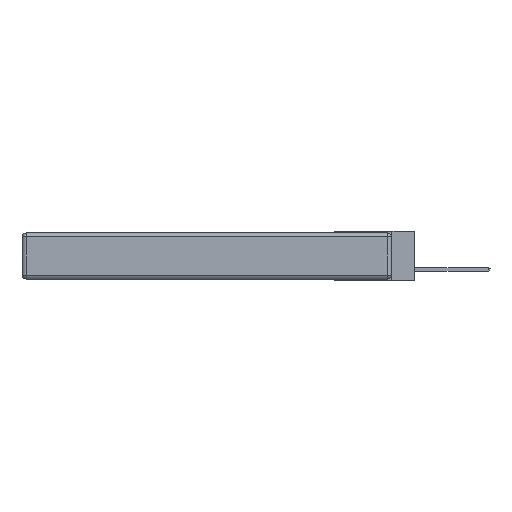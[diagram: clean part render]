
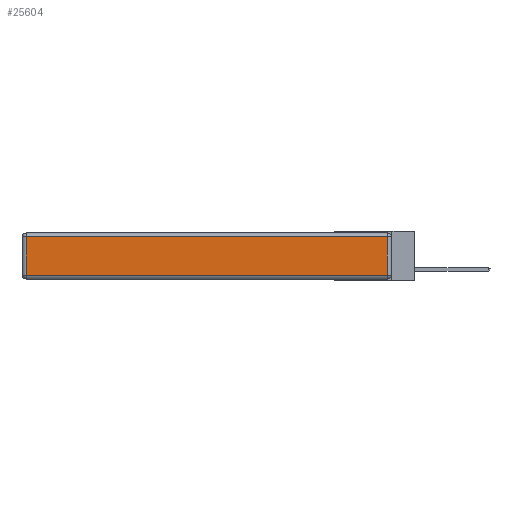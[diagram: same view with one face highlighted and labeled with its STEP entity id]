
A CAD part, left-side view. The second image highlights one B-rep face of the part: STEP entity #25604.
In plain terms, the highlighted planar face has unit normal (-1, 0, 0).
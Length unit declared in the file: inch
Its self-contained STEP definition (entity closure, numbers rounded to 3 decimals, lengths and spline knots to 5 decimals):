
#235 = VECTOR ( 'NONE', #12016, 39.37008 ) ;
#1295 = LINE ( 'NONE', #10112, #29966 ) ;
#2173 = VERTEX_POINT ( 'NONE', #31284 ) ;
#2407 = AXIS2_PLACEMENT_3D ( 'NONE', #12911, #10444, #15293 ) ;
#3053 = EDGE_CURVE ( 'NONE', #2173, #26531, #12572, .T. ) ;
#6768 = VERTEX_POINT ( 'NONE', #28451 ) ;
#9256 = LINE ( 'NONE', #20944, #17647 ) ;
#10112 = CARTESIAN_POINT ( 'NONE',  ( 0., 2.75, -0.03 ) ) ;
#10444 = DIRECTION ( 'NONE',  ( -1., 0., 0. ) ) ;
#10727 = ORIENTED_EDGE ( 'NONE', *, *, #3053, .T. ) ;
#10991 = LINE ( 'NONE', #29425, #235 ) ;
#11789 = ORIENTED_EDGE ( 'NONE', *, *, #19651, .T. ) ;
#12016 = DIRECTION ( 'NONE',  ( 0., 0., 1. ) ) ;
#12572 = LINE ( 'NONE', #29220, #16759 ) ;
#12911 = CARTESIAN_POINT ( 'NONE',  ( 0., 0., -0.343 ) ) ;
#15293 = DIRECTION ( 'NONE',  ( 0., 0., 1. ) ) ;
#16759 = VECTOR ( 'NONE', #16890, 39.37008 ) ;
#16890 = DIRECTION ( 'NONE',  ( 0., -1., 0. ) ) ;
#17482 = DIRECTION ( 'NONE',  ( 0., 1., 0. ) ) ;
#17647 = VECTOR ( 'NONE', #23733, 39.37008 ) ;
#19651 = EDGE_CURVE ( 'NONE', #6768, #23016, #1295, .T. ) ;
#19965 = EDGE_LOOP ( 'NONE', ( #10727, #23942, #11789, #30455 ) ) ;
#20638 = EDGE_CURVE ( 'NONE', #23016, #2173, #9256, .T. ) ;
#20944 = CARTESIAN_POINT ( 'NONE',  ( 0., 2.72, -0.343 ) ) ;
#22236 = FACE_OUTER_BOUND ( 'NONE', #19965, .T. ) ;
#23016 = VERTEX_POINT ( 'NONE', #29051 ) ;
#23733 = DIRECTION ( 'NONE',  ( 0., 0., -1. ) ) ;
#23942 = ORIENTED_EDGE ( 'NONE', *, *, #30385, .T. ) ;
#25079 = PLANE ( 'NONE',  #2407 ) ;
#25604 = ADVANCED_FACE ( 'NONE', ( #22236 ), #25079, .T. ) ;
#26531 = VERTEX_POINT ( 'NONE', #30889 ) ;
#28451 = CARTESIAN_POINT ( 'NONE',  ( 0., 0.03, -0.03 ) ) ;
#29051 = CARTESIAN_POINT ( 'NONE',  ( 0., 2.72, -0.03 ) ) ;
#29220 = CARTESIAN_POINT ( 'NONE',  ( 0., 0., -0.313 ) ) ;
#29425 = CARTESIAN_POINT ( 'NONE',  ( 0., 0.03, -0.343 ) ) ;
#29966 = VECTOR ( 'NONE', #17482, 39.37008 ) ;
#30385 = EDGE_CURVE ( 'NONE', #26531, #6768, #10991, .T. ) ;
#30455 = ORIENTED_EDGE ( 'NONE', *, *, #20638, .T. ) ;
#30889 = CARTESIAN_POINT ( 'NONE',  ( 0., 0.03, -0.313 ) ) ;
#31284 = CARTESIAN_POINT ( 'NONE',  ( 0., 2.72, -0.313 ) ) ;
